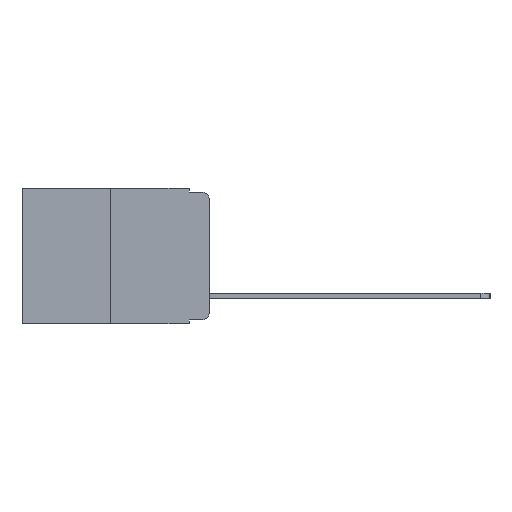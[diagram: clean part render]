
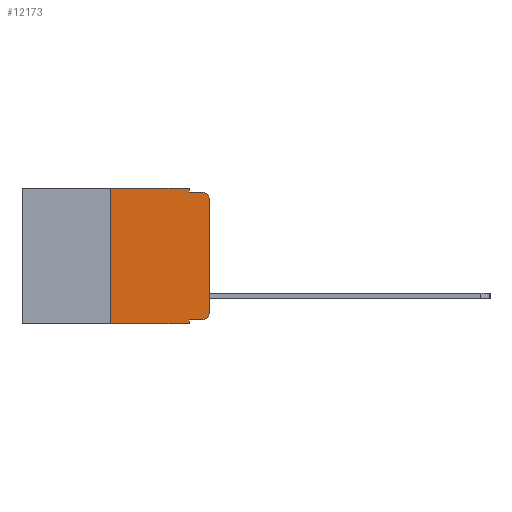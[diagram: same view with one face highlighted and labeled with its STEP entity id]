
A CAD part, left-side view. The second image highlights one B-rep face of the part: STEP entity #12173.
In plain terms, the highlighted planar face has unit normal (-1, 0, 0).
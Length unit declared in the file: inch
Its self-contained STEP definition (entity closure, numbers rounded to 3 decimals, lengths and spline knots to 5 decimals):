
#172 = DIRECTION ( 'NONE',  ( 0., 0., -1. ) ) ;
#373 = CARTESIAN_POINT ( 'NONE',  ( 0., 0.25, 0. ) ) ;
#429 = CARTESIAN_POINT ( 'NONE',  ( 0., 0.051, -0.343 ) ) ;
#433 = ORIENTED_EDGE ( 'NONE', *, *, #3895, .T. ) ;
#817 = PLANE ( 'NONE',  #11016 ) ;
#1466 = VERTEX_POINT ( 'NONE', #9732 ) ;
#1605 = VECTOR ( 'NONE', #12162, 39.37008 ) ;
#1755 = CIRCLE ( 'NONE', #8193, 0.02 ) ;
#1880 = DIRECTION ( 'NONE',  ( 0., -1., 0. ) ) ;
#1914 = EDGE_CURVE ( 'NONE', #1466, #2820, #12029, .T. ) ;
#2368 = CARTESIAN_POINT ( 'NONE',  ( 0., 0.25, 0. ) ) ;
#2737 = VECTOR ( 'NONE', #6928, 39.37008 ) ;
#2767 = DIRECTION ( 'NONE',  ( 0., -1., 0. ) ) ;
#2820 = VERTEX_POINT ( 'NONE', #8576 ) ;
#3196 = VERTEX_POINT ( 'NONE', #429 ) ;
#3385 = DIRECTION ( 'NONE',  ( 0., 0., -1. ) ) ;
#3411 = DIRECTION ( 'NONE',  ( -1., 0., 0. ) ) ;
#3413 = CARTESIAN_POINT ( 'NONE',  ( 0., 0.02, -0.313 ) ) ;
#3443 = CARTESIAN_POINT ( 'NONE',  ( 0., 0.02, -0.03 ) ) ;
#3638 = CARTESIAN_POINT ( 'NONE',  ( 0., 0.051, -0.01 ) ) ;
#3741 = LINE ( 'NONE', #9152, #9382 ) ;
#3895 = EDGE_CURVE ( 'NONE', #2820, #5331, #4140, .T. ) ;
#3938 = VECTOR ( 'NONE', #1880, 39.37008 ) ;
#4024 = CARTESIAN_POINT ( 'NONE',  ( 0., 0.051, -0.333 ) ) ;
#4043 = DIRECTION ( 'NONE',  ( 0., -1., 0. ) ) ;
#4082 = DIRECTION ( 'NONE',  ( 1., 0., 0. ) ) ;
#4140 = LINE ( 'NONE', #12357, #1605 ) ;
#4531 = DIRECTION ( 'NONE',  ( 0., 0., -1. ) ) ;
#4539 = CARTESIAN_POINT ( 'NONE',  ( 0., 0.051, 0. ) ) ;
#4548 = ORIENTED_EDGE ( 'NONE', *, *, #5180, .T. ) ;
#4580 = CARTESIAN_POINT ( 'NONE',  ( 0., 0.051, -0.01 ) ) ;
#4873 = EDGE_CURVE ( 'NONE', #11595, #1466, #12327, .T. ) ;
#5108 = CARTESIAN_POINT ( 'NONE',  ( 0., 0.473, 0. ) ) ;
#5120 = VERTEX_POINT ( 'NONE', #3638 ) ;
#5180 = EDGE_CURVE ( 'NONE', #5931, #3196, #11170, .T. ) ;
#5188 = ORIENTED_EDGE ( 'NONE', *, *, #8966, .F. ) ;
#5260 = EDGE_CURVE ( 'NONE', #6268, #5120, #7805, .T. ) ;
#5331 = VERTEX_POINT ( 'NONE', #7413 ) ;
#5503 = ORIENTED_EDGE ( 'NONE', *, *, #9722, .F. ) ;
#5819 = AXIS2_PLACEMENT_3D ( 'NONE', #3413, #3411, #3385 ) ;
#5913 = VECTOR ( 'NONE', #7742, 39.37008 ) ;
#5931 = VERTEX_POINT ( 'NONE', #13122 ) ;
#6268 = VERTEX_POINT ( 'NONE', #6943 ) ;
#6274 = CARTESIAN_POINT ( 'NONE',  ( 0., 0.051, -0.333 ) ) ;
#6928 = DIRECTION ( 'NONE',  ( 0., -1., 0. ) ) ;
#6943 = CARTESIAN_POINT ( 'NONE',  ( 0., 0.051, 0. ) ) ;
#7011 = EDGE_CURVE ( 'NONE', #5120, #11557, #10978, .T. ) ;
#7413 = CARTESIAN_POINT ( 'NONE',  ( 0., 0., -0.03 ) ) ;
#7460 = VECTOR ( 'NONE', #12918, 39.37008 ) ;
#7695 = EDGE_CURVE ( 'NONE', #11595, #3196, #7749, .T. ) ;
#7742 = DIRECTION ( 'NONE',  ( 0., 0., 1. ) ) ;
#7749 = LINE ( 'NONE', #4539, #10798 ) ;
#7805 = LINE ( 'NONE', #13119, #7460 ) ;
#8193 = AXIS2_PLACEMENT_3D ( 'NONE', #3443, #10816, #4531 ) ;
#8405 = CARTESIAN_POINT ( 'NONE',  ( 0., 0.02, -0.01 ) ) ;
#8576 = CARTESIAN_POINT ( 'NONE',  ( 0., 0., -0.313 ) ) ;
#8966 = EDGE_CURVE ( 'NONE', #5931, #10712, #11497, .T. ) ;
#9152 = CARTESIAN_POINT ( 'NONE',  ( 0., 0.473, 0. ) ) ;
#9297 = CARTESIAN_POINT ( 'NONE',  ( 0., 0.473, -0.343 ) ) ;
#9382 = VECTOR ( 'NONE', #2767, 39.37008 ) ;
#9687 = ORIENTED_EDGE ( 'NONE', *, *, #7695, .F. ) ;
#9722 = EDGE_CURVE ( 'NONE', #10712, #6268, #3741, .T. ) ;
#9732 = CARTESIAN_POINT ( 'NONE',  ( 0., 0.02, -0.333 ) ) ;
#9965 = ORIENTED_EDGE ( 'NONE', *, *, #13001, .T. ) ;
#10190 = EDGE_LOOP ( 'NONE', ( #433, #9965, #11573, #13068, #5503, #5188, #4548, #9687, #11960, #13274 ) ) ;
#10712 = VERTEX_POINT ( 'NONE', #373 ) ;
#10798 = VECTOR ( 'NONE', #172, 39.37008 ) ;
#10816 = DIRECTION ( 'NONE',  ( -1., 0., 0. ) ) ;
#10978 = LINE ( 'NONE', #4580, #13110 ) ;
#11016 = AXIS2_PLACEMENT_3D ( 'NONE', #5108, #4082, #11442 ) ;
#11170 = LINE ( 'NONE', #9297, #2737 ) ;
#11442 = DIRECTION ( 'NONE',  ( 0., 0., -1. ) ) ;
#11497 = LINE ( 'NONE', #2368, #5913 ) ;
#11557 = VERTEX_POINT ( 'NONE', #8405 ) ;
#11573 = ORIENTED_EDGE ( 'NONE', *, *, #7011, .F. ) ;
#11595 = VERTEX_POINT ( 'NONE', #6274 ) ;
#11960 = ORIENTED_EDGE ( 'NONE', *, *, #4873, .T. ) ;
#12029 = CIRCLE ( 'NONE', #5819, 0.02 ) ;
#12162 = DIRECTION ( 'NONE',  ( 0., 0., 1. ) ) ;
#12173 = ADVANCED_FACE ( 'NONE', ( #12374 ), #817, .F. ) ;
#12327 = LINE ( 'NONE', #4024, #3938 ) ;
#12357 = CARTESIAN_POINT ( 'NONE',  ( 0., 0., 0. ) ) ;
#12374 = FACE_OUTER_BOUND ( 'NONE', #10190, .T. ) ;
#12918 = DIRECTION ( 'NONE',  ( 0., 0., -1. ) ) ;
#13001 = EDGE_CURVE ( 'NONE', #5331, #11557, #1755, .T. ) ;
#13068 = ORIENTED_EDGE ( 'NONE', *, *, #5260, .F. ) ;
#13110 = VECTOR ( 'NONE', #4043, 39.37008 ) ;
#13119 = CARTESIAN_POINT ( 'NONE',  ( 0., 0.051, 0. ) ) ;
#13122 = CARTESIAN_POINT ( 'NONE',  ( 0., 0.25, -0.343 ) ) ;
#13274 = ORIENTED_EDGE ( 'NONE', *, *, #1914, .T. ) ;
